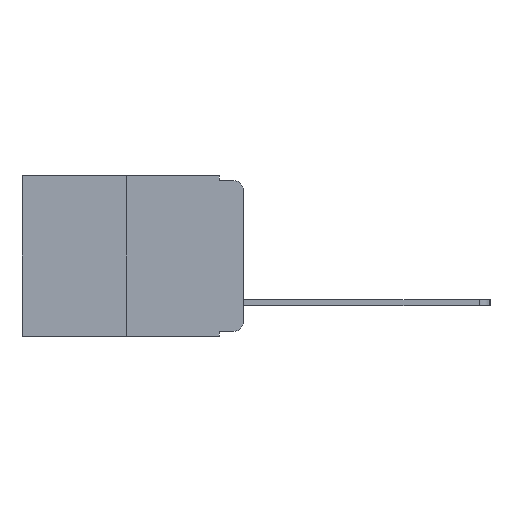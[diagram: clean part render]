
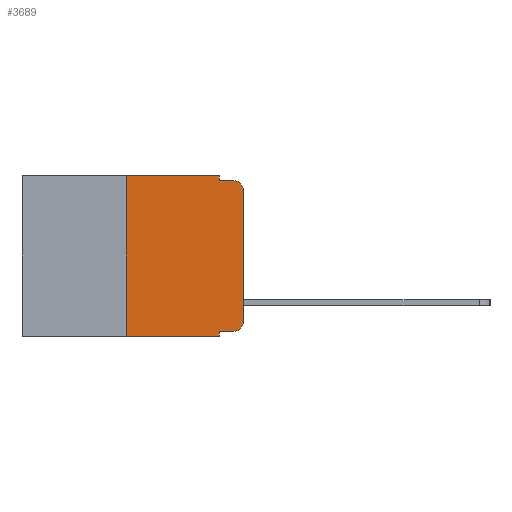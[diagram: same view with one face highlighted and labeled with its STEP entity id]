
A CAD part, left-side view. The second image highlights one B-rep face of the part: STEP entity #3689.
In plain terms, the highlighted planar face has unit normal (-1, 0, 0).
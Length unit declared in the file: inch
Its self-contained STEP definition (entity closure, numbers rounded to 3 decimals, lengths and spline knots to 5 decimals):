
#18 = ORIENTED_EDGE ( 'NONE', *, *, #5932, .T. ) ;
#97 = CARTESIAN_POINT ( 'NONE',  ( 0., 0.473, 0. ) ) ;
#187 = VERTEX_POINT ( 'NONE', #7143 ) ;
#269 = CARTESIAN_POINT ( 'NONE',  ( 0., 0.25, 0. ) ) ;
#367 = ORIENTED_EDGE ( 'NONE', *, *, #8613, .T. ) ;
#708 = CARTESIAN_POINT ( 'NONE',  ( 0., 0.02, -0.333 ) ) ;
#853 = DIRECTION ( 'NONE',  ( 0., 0., -1. ) ) ;
#940 = VERTEX_POINT ( 'NONE', #12213 ) ;
#1011 = DIRECTION ( 'NONE',  ( 0., -1., 0. ) ) ;
#1121 = LINE ( 'NONE', #9281, #8609 ) ;
#1200 = VERTEX_POINT ( 'NONE', #8261 ) ;
#1310 = EDGE_LOOP ( 'NONE', ( #3411, #3892, #4402, #5974, #6329, #8543, #8881, #11374, #18, #367 ) ) ;
#1613 = VERTEX_POINT ( 'NONE', #10245 ) ;
#1790 = CARTESIAN_POINT ( 'NONE',  ( 0., 0.051, -0.01 ) ) ;
#1867 = CIRCLE ( 'NONE', #7511, 0.02 ) ;
#2295 = AXIS2_PLACEMENT_3D ( 'NONE', #97, #6909, #5247 ) ;
#2475 = EDGE_CURVE ( 'NONE', #940, #1200, #10015, .T. ) ;
#2533 = CARTESIAN_POINT ( 'NONE',  ( 0., 0.473, 0. ) ) ;
#2817 = EDGE_CURVE ( 'NONE', #1613, #7571, #9440, .T. ) ;
#2854 = EDGE_CURVE ( 'NONE', #7571, #1200, #1867, .T. ) ;
#2864 = VERTEX_POINT ( 'NONE', #4972 ) ;
#2865 = LINE ( 'NONE', #9456, #11656 ) ;
#3411 = ORIENTED_EDGE ( 'NONE', *, *, #2817, .T. ) ;
#3495 = CARTESIAN_POINT ( 'NONE',  ( 0., 0.02, -0.03 ) ) ;
#3689 = ADVANCED_FACE ( 'NONE', ( #9705 ), #4507, .F. ) ;
#3741 = LINE ( 'NONE', #3897, #10987 ) ;
#3773 = CARTESIAN_POINT ( 'NONE',  ( 0., 0.02, -0.313 ) ) ;
#3892 = ORIENTED_EDGE ( 'NONE', *, *, #2854, .T. ) ;
#3897 = CARTESIAN_POINT ( 'NONE',  ( 0., 0.25, 0. ) ) ;
#3910 = DIRECTION ( 'NONE',  ( 0., 0., -1. ) ) ;
#4015 = VERTEX_POINT ( 'NONE', #10627 ) ;
#4018 = VERTEX_POINT ( 'NONE', #269 ) ;
#4402 = ORIENTED_EDGE ( 'NONE', *, *, #2475, .F. ) ;
#4507 = PLANE ( 'NONE',  #2295 ) ;
#4555 = VECTOR ( 'NONE', #11625, 39.37008 ) ;
#4604 = EDGE_CURVE ( 'NONE', #2864, #940, #1121, .T. ) ;
#4706 = DIRECTION ( 'NONE',  ( 0., 0., -1. ) ) ;
#4972 = CARTESIAN_POINT ( 'NONE',  ( 0., 0.051, 0. ) ) ;
#5247 = DIRECTION ( 'NONE',  ( 0., 0., -1. ) ) ;
#5354 = LINE ( 'NONE', #6990, #7302 ) ;
#5696 = DIRECTION ( 'NONE',  ( 0., 0., -1. ) ) ;
#5932 = EDGE_CURVE ( 'NONE', #7269, #10746, #5354, .T. ) ;
#5974 = ORIENTED_EDGE ( 'NONE', *, *, #4604, .F. ) ;
#6074 = LINE ( 'NONE', #7133, #8274 ) ;
#6329 = ORIENTED_EDGE ( 'NONE', *, *, #9789, .F. ) ;
#6485 = EDGE_CURVE ( 'NONE', #7269, #187, #2865, .T. ) ;
#6909 = DIRECTION ( 'NONE',  ( 1., 0., 0. ) ) ;
#6990 = CARTESIAN_POINT ( 'NONE',  ( 0., 0.051, -0.333 ) ) ;
#7129 = EDGE_CURVE ( 'NONE', #4015, #4018, #3741, .T. ) ;
#7133 = CARTESIAN_POINT ( 'NONE',  ( 0., 0.473, -0.343 ) ) ;
#7143 = CARTESIAN_POINT ( 'NONE',  ( 0., 0.051, -0.343 ) ) ;
#7269 = VERTEX_POINT ( 'NONE', #8688 ) ;
#7296 = VECTOR ( 'NONE', #8182, 39.37008 ) ;
#7302 = VECTOR ( 'NONE', #1011, 39.37008 ) ;
#7511 = AXIS2_PLACEMENT_3D ( 'NONE', #3495, #9038, #5696 ) ;
#7571 = VERTEX_POINT ( 'NONE', #9058 ) ;
#8182 = DIRECTION ( 'NONE',  ( 0., -1., 0. ) ) ;
#8261 = CARTESIAN_POINT ( 'NONE',  ( 0., 0.02, -0.01 ) ) ;
#8274 = VECTOR ( 'NONE', #9835, 39.37008 ) ;
#8317 = DIRECTION ( 'NONE',  ( 0., -1., 0. ) ) ;
#8543 = ORIENTED_EDGE ( 'NONE', *, *, #7129, .F. ) ;
#8609 = VECTOR ( 'NONE', #853, 39.37008 ) ;
#8613 = EDGE_CURVE ( 'NONE', #10746, #1613, #11406, .T. ) ;
#8688 = CARTESIAN_POINT ( 'NONE',  ( 0., 0.051, -0.333 ) ) ;
#8881 = ORIENTED_EDGE ( 'NONE', *, *, #10358, .T. ) ;
#9038 = DIRECTION ( 'NONE',  ( -1., 0., 0. ) ) ;
#9058 = CARTESIAN_POINT ( 'NONE',  ( 0., 0., -0.03 ) ) ;
#9281 = CARTESIAN_POINT ( 'NONE',  ( 0., 0.051, 0. ) ) ;
#9440 = LINE ( 'NONE', #9806, #4555 ) ;
#9456 = CARTESIAN_POINT ( 'NONE',  ( 0., 0.051, 0. ) ) ;
#9705 = FACE_OUTER_BOUND ( 'NONE', #1310, .T. ) ;
#9789 = EDGE_CURVE ( 'NONE', #4018, #2864, #11398, .T. ) ;
#9806 = CARTESIAN_POINT ( 'NONE',  ( 0., 0., 0. ) ) ;
#9835 = DIRECTION ( 'NONE',  ( 0., -1., 0. ) ) ;
#9853 = AXIS2_PLACEMENT_3D ( 'NONE', #3773, #10188, #4706 ) ;
#10015 = LINE ( 'NONE', #1790, #11999 ) ;
#10188 = DIRECTION ( 'NONE',  ( -1., 0., 0. ) ) ;
#10245 = CARTESIAN_POINT ( 'NONE',  ( 0., 0., -0.313 ) ) ;
#10287 = DIRECTION ( 'NONE',  ( 0., 0., 1. ) ) ;
#10358 = EDGE_CURVE ( 'NONE', #4015, #187, #6074, .T. ) ;
#10627 = CARTESIAN_POINT ( 'NONE',  ( 0., 0.25, -0.343 ) ) ;
#10746 = VERTEX_POINT ( 'NONE', #708 ) ;
#10987 = VECTOR ( 'NONE', #10287, 39.37008 ) ;
#11374 = ORIENTED_EDGE ( 'NONE', *, *, #6485, .F. ) ;
#11398 = LINE ( 'NONE', #2533, #7296 ) ;
#11406 = CIRCLE ( 'NONE', #9853, 0.02 ) ;
#11625 = DIRECTION ( 'NONE',  ( 0., 0., 1. ) ) ;
#11656 = VECTOR ( 'NONE', #3910, 39.37008 ) ;
#11999 = VECTOR ( 'NONE', #8317, 39.37008 ) ;
#12213 = CARTESIAN_POINT ( 'NONE',  ( 0., 0.051, -0.01 ) ) ;
